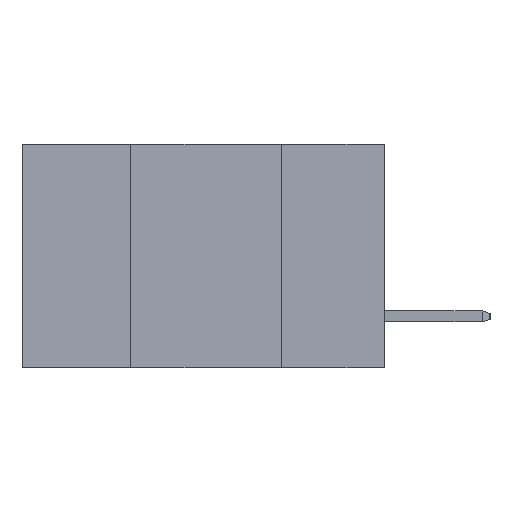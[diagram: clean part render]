
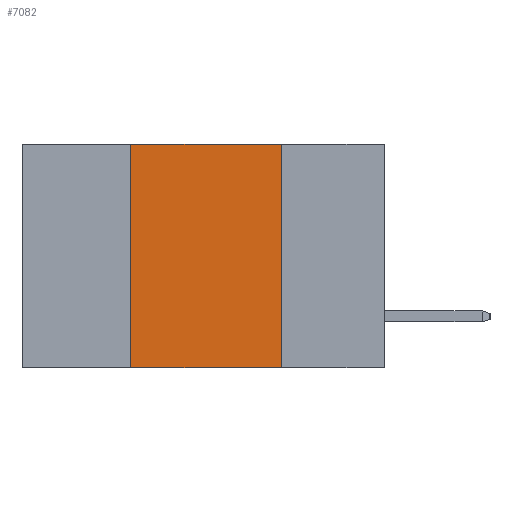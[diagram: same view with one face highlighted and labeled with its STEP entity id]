
A CAD part, left-side view. The second image highlights one B-rep face of the part: STEP entity #7082.
In plain terms, the highlighted planar face has unit normal (-1, 0, 0).
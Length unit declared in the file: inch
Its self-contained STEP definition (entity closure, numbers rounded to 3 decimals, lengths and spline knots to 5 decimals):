
#900 = CARTESIAN_POINT ( 'NONE',  ( 0., 0.17, 0. ) ) ;
#1358 = ORIENTED_EDGE ( 'NONE', *, *, #5844, .F. ) ;
#1491 = VERTEX_POINT ( 'NONE', #3316 ) ;
#1699 = VECTOR ( 'NONE', #10167, 39.37008 ) ;
#1970 = EDGE_CURVE ( 'NONE', #1491, #12264, #9712, .T. ) ;
#2104 = FACE_OUTER_BOUND ( 'NONE', #8523, .T. ) ;
#2149 = ORIENTED_EDGE ( 'NONE', *, *, #13359, .F. ) ;
#2372 = CARTESIAN_POINT ( 'NONE',  ( 0., 0.17, 0. ) ) ;
#2434 = EDGE_CURVE ( 'NONE', #6589, #13046, #12073, .T. ) ;
#2649 = VECTOR ( 'NONE', #8402, 39.37008 ) ;
#3244 = DIRECTION ( 'NONE',  ( 0., -1., 0. ) ) ;
#3316 = CARTESIAN_POINT ( 'NONE',  ( 0., 0.42, -0.37 ) ) ;
#4086 = DIRECTION ( 'NONE',  ( 0., -1., 0. ) ) ;
#4109 = PLANE ( 'NONE',  #10055 ) ;
#4600 = VECTOR ( 'NONE', #3244, 39.37008 ) ;
#4649 = LINE ( 'NONE', #11189, #1699 ) ;
#5844 = EDGE_CURVE ( 'NONE', #13046, #12264, #10630, .T. ) ;
#6060 = ORIENTED_EDGE ( 'NONE', *, *, #1970, .T. ) ;
#6256 = DIRECTION ( 'NONE',  ( 1., 0., 0. ) ) ;
#6441 = CARTESIAN_POINT ( 'NONE',  ( 0., 0.42, 0. ) ) ;
#6589 = VERTEX_POINT ( 'NONE', #6441 ) ;
#7082 = ADVANCED_FACE ( 'NONE', ( #2104 ), #4109, .F. ) ;
#8217 = CARTESIAN_POINT ( 'NONE',  ( 0., 0.6, 0. ) ) ;
#8402 = DIRECTION ( 'NONE',  ( 0., 0., -1. ) ) ;
#8497 = CARTESIAN_POINT ( 'NONE',  ( 0., 0.6, -0.37 ) ) ;
#8523 = EDGE_LOOP ( 'NONE', ( #1358, #12302, #2149, #6060 ) ) ;
#9701 = VECTOR ( 'NONE', #4086, 39.37008 ) ;
#9712 = LINE ( 'NONE', #8497, #4600 ) ;
#10055 = AXIS2_PLACEMENT_3D ( 'NONE', #12283, #6256, #13284 ) ;
#10167 = DIRECTION ( 'NONE',  ( 0., 0., 1. ) ) ;
#10630 = LINE ( 'NONE', #900, #2649 ) ;
#11189 = CARTESIAN_POINT ( 'NONE',  ( 0., 0.42, 0. ) ) ;
#12073 = LINE ( 'NONE', #8217, #9701 ) ;
#12264 = VERTEX_POINT ( 'NONE', #13471 ) ;
#12283 = CARTESIAN_POINT ( 'NONE',  ( 0., 0.6, 0. ) ) ;
#12302 = ORIENTED_EDGE ( 'NONE', *, *, #2434, .F. ) ;
#13046 = VERTEX_POINT ( 'NONE', #2372 ) ;
#13284 = DIRECTION ( 'NONE',  ( 0., 0., -1. ) ) ;
#13359 = EDGE_CURVE ( 'NONE', #1491, #6589, #4649, .T. ) ;
#13471 = CARTESIAN_POINT ( 'NONE',  ( 0., 0.17, -0.37 ) ) ;
